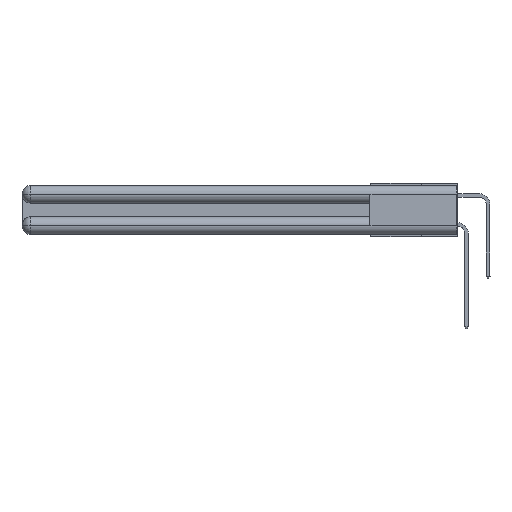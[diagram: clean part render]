
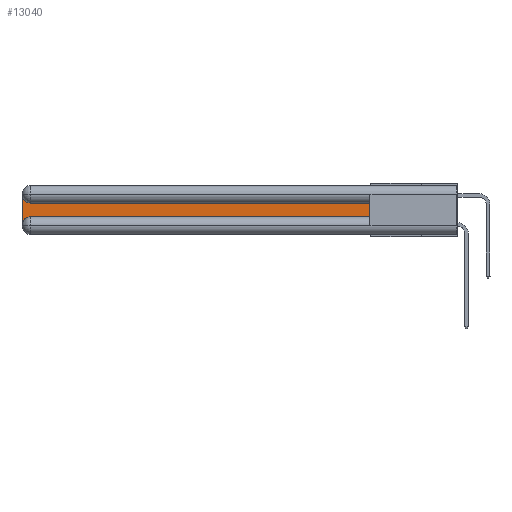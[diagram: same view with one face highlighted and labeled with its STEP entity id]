
A CAD part, left-side view. The second image highlights one B-rep face of the part: STEP entity #13040.
In plain terms, the highlighted planar face has unit normal (-1, 0, 0).
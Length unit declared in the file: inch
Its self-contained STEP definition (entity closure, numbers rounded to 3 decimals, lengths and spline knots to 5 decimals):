
#1133 = CARTESIAN_POINT ( 'NONE',  ( 0.075, 3., -0.0625 ) ) ;
#1387 = CARTESIAN_POINT ( 'NONE',  ( 0.075, 2.94, -0.0625 ) ) ;
#1501 = VERTEX_POINT ( 'NONE', #2543 ) ;
#1839 = CARTESIAN_POINT ( 'NONE',  ( 0.075, 3., -0.2775 ) ) ;
#2154 = CARTESIAN_POINT ( 'NONE',  ( 0.075, 3., -0.2175 ) ) ;
#2543 = CARTESIAN_POINT ( 'NONE',  ( 0.075, 0.6, -0.2175 ) ) ;
#3183 = CIRCLE ( 'NONE', #8316, 0.06 ) ;
#4609 = VECTOR ( 'NONE', #5945, 39.37008 ) ;
#4789 = VECTOR ( 'NONE', #18736, 39.37008 ) ;
#5293 = DIRECTION ( 'NONE',  ( 1., 0., 0. ) ) ;
#5945 = DIRECTION ( 'NONE',  ( 0., -1., 0. ) ) ;
#6237 = DIRECTION ( 'NONE',  ( 0., 1., 0. ) ) ;
#6979 = PLANE ( 'NONE',  #26265 ) ;
#7209 = VERTEX_POINT ( 'NONE', #18635 ) ;
#7679 = VERTEX_POINT ( 'NONE', #1133 ) ;
#8316 = AXIS2_PLACEMENT_3D ( 'NONE', #1387, #30743, #9153 ) ;
#9153 = DIRECTION ( 'NONE',  ( 0., 0., -1. ) ) ;
#9663 = CARTESIAN_POINT ( 'NONE',  ( 0.075, 2.94, -0.2775 ) ) ;
#9818 = AXIS2_PLACEMENT_3D ( 'NONE', #9663, #12398, #31138 ) ;
#9963 = EDGE_LOOP ( 'NONE', ( #32116, #10529, #31041, #33366, #14676, #24536 ) ) ;
#10355 = VERTEX_POINT ( 'NONE', #17052 ) ;
#10529 = ORIENTED_EDGE ( 'NONE', *, *, #14608, .T. ) ;
#10877 = EDGE_CURVE ( 'NONE', #17633, #13851, #12768, .T. ) ;
#11866 = VECTOR ( 'NONE', #21063, 39.37008 ) ;
#12398 = DIRECTION ( 'NONE',  ( 1., 0., 0. ) ) ;
#12768 = CIRCLE ( 'NONE', #9818, 0.06 ) ;
#13040 = ADVANCED_FACE ( 'NONE', ( #16665 ), #6979, .F. ) ;
#13651 = CARTESIAN_POINT ( 'NONE',  ( 0.075, 0.6, -0.2175 ) ) ;
#13851 = VERTEX_POINT ( 'NONE', #32167 ) ;
#14608 = EDGE_CURVE ( 'NONE', #7209, #7679, #3183, .T. ) ;
#14676 = ORIENTED_EDGE ( 'NONE', *, *, #33406, .T. ) ;
#16665 = FACE_OUTER_BOUND ( 'NONE', #9963, .T. ) ;
#17052 = CARTESIAN_POINT ( 'NONE',  ( 0.075, 0.6, -0.1225 ) ) ;
#17633 = VERTEX_POINT ( 'NONE', #1839 ) ;
#18635 = CARTESIAN_POINT ( 'NONE',  ( 0.075, 2.94, -0.1225 ) ) ;
#18736 = DIRECTION ( 'NONE',  ( 0., 0., -1. ) ) ;
#18888 = LINE ( 'NONE', #29940, #29047 ) ;
#21063 = DIRECTION ( 'NONE',  ( 0., 0., 1. ) ) ;
#22390 = LINE ( 'NONE', #13651, #4609 ) ;
#22534 = LINE ( 'NONE', #34298, #11866 ) ;
#22572 = EDGE_CURVE ( 'NONE', #7679, #17633, #31915, .T. ) ;
#24536 = ORIENTED_EDGE ( 'NONE', *, *, #31778, .T. ) ;
#24937 = EDGE_CURVE ( 'NONE', #10355, #7209, #18888, .T. ) ;
#26265 = AXIS2_PLACEMENT_3D ( 'NONE', #26872, #5293, #34771 ) ;
#26872 = CARTESIAN_POINT ( 'NONE',  ( 0.075, 3., -0.1225 ) ) ;
#29047 = VECTOR ( 'NONE', #6237, 39.37008 ) ;
#29940 = CARTESIAN_POINT ( 'NONE',  ( 0.075, 0.6, -0.1225 ) ) ;
#30743 = DIRECTION ( 'NONE',  ( 1., 0., 0. ) ) ;
#31041 = ORIENTED_EDGE ( 'NONE', *, *, #22572, .T. ) ;
#31138 = DIRECTION ( 'NONE',  ( 0., 0., -1. ) ) ;
#31778 = EDGE_CURVE ( 'NONE', #1501, #10355, #22534, .T. ) ;
#31915 = LINE ( 'NONE', #2154, #4789 ) ;
#32116 = ORIENTED_EDGE ( 'NONE', *, *, #24937, .T. ) ;
#32167 = CARTESIAN_POINT ( 'NONE',  ( 0.075, 2.94, -0.2175 ) ) ;
#33366 = ORIENTED_EDGE ( 'NONE', *, *, #10877, .T. ) ;
#33406 = EDGE_CURVE ( 'NONE', #13851, #1501, #22390, .T. ) ;
#34298 = CARTESIAN_POINT ( 'NONE',  ( 0.075, 0.6, -0.2175 ) ) ;
#34771 = DIRECTION ( 'NONE',  ( 0., 0., -1. ) ) ;
